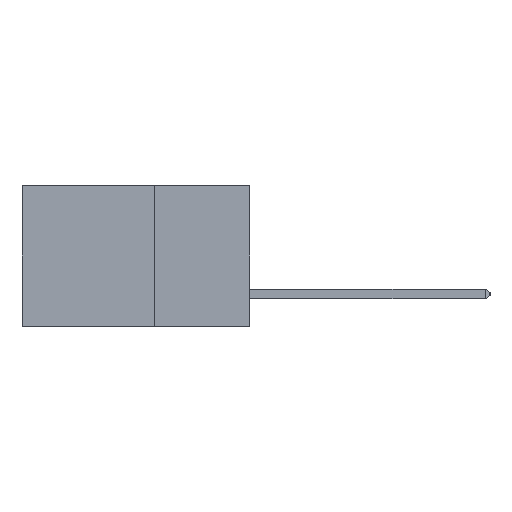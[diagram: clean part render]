
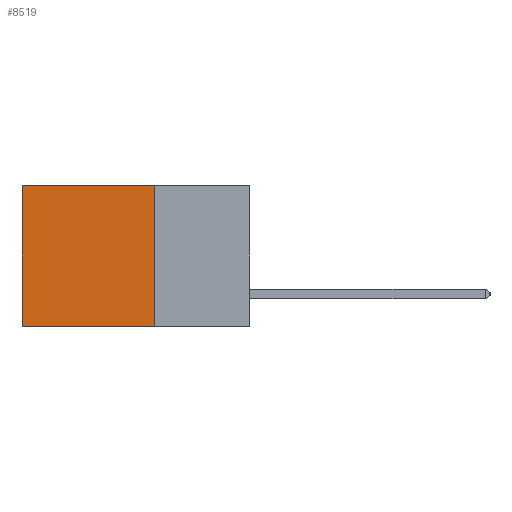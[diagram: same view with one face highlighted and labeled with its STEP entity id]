
A CAD part, left-side view. The second image highlights one B-rep face of the part: STEP entity #8519.
In plain terms, the highlighted planar face has unit normal (-1, 0, 0).
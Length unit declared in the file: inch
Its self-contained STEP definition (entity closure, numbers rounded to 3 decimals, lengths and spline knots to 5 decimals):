
#1531 = DIRECTION ( 'NONE',  ( 0., 0., -1. ) ) ;
#2820 = ORIENTED_EDGE ( 'NONE', *, *, #31856, .T. ) ;
#3117 = DIRECTION ( 'NONE',  ( 0., 1., 0. ) ) ;
#3577 = LINE ( 'NONE', #36829, #6129 ) ;
#3712 = DIRECTION ( 'NONE',  ( 0., 0., -1. ) ) ;
#5119 = DIRECTION ( 'NONE',  ( 0., 0., -1. ) ) ;
#5290 = EDGE_CURVE ( 'NONE', #38703, #34493, #7250, .T. ) ;
#6129 = VECTOR ( 'NONE', #32997, 39.37008 ) ;
#6438 = VERTEX_POINT ( 'NONE', #40004 ) ;
#7250 = LINE ( 'NONE', #19268, #40865 ) ;
#8394 = CARTESIAN_POINT ( 'NONE',  ( 0.2875, 0.6, 0. ) ) ;
#8519 = ADVANCED_FACE ( 'NONE', ( #40928 ), #27375, .F. ) ;
#10884 = VECTOR ( 'NONE', #3712, 39.37008 ) ;
#11191 = CARTESIAN_POINT ( 'NONE',  ( 0.2875, 0.25, 0. ) ) ;
#12404 = LINE ( 'NONE', #36567, #10884 ) ;
#15074 = EDGE_CURVE ( 'NONE', #6438, #39119, #3577, .T. ) ;
#15323 = LINE ( 'NONE', #24394, #40306 ) ;
#19268 = CARTESIAN_POINT ( 'NONE',  ( 0.2875, 0.25, -0.37 ) ) ;
#24394 = CARTESIAN_POINT ( 'NONE',  ( 0.2875, 0.6, 0. ) ) ;
#25441 = CARTESIAN_POINT ( 'NONE',  ( 0.2875, 0.25, -0.37 ) ) ;
#26002 = ORIENTED_EDGE ( 'NONE', *, *, #15074, .T. ) ;
#27375 = PLANE ( 'NONE',  #34944 ) ;
#31313 = CARTESIAN_POINT ( 'NONE',  ( 0.2875, 0.6, -0.37 ) ) ;
#31856 = EDGE_CURVE ( 'NONE', #39119, #34493, #15323, .T. ) ;
#32197 = ORIENTED_EDGE ( 'NONE', *, *, #5290, .F. ) ;
#32997 = DIRECTION ( 'NONE',  ( 0., 1., 0. ) ) ;
#34493 = VERTEX_POINT ( 'NONE', #31313 ) ;
#34944 = AXIS2_PLACEMENT_3D ( 'NONE', #11191, #40506, #1531 ) ;
#36282 = EDGE_CURVE ( 'NONE', #6438, #38703, #12404, .T. ) ;
#36481 = EDGE_LOOP ( 'NONE', ( #2820, #32197, #39844, #26002 ) ) ;
#36567 = CARTESIAN_POINT ( 'NONE',  ( 0.2875, 0.25, 0. ) ) ;
#36829 = CARTESIAN_POINT ( 'NONE',  ( 0.2875, 0.25, 0. ) ) ;
#38703 = VERTEX_POINT ( 'NONE', #25441 ) ;
#39119 = VERTEX_POINT ( 'NONE', #8394 ) ;
#39844 = ORIENTED_EDGE ( 'NONE', *, *, #36282, .F. ) ;
#40004 = CARTESIAN_POINT ( 'NONE',  ( 0.2875, 0.25, 0. ) ) ;
#40306 = VECTOR ( 'NONE', #5119, 39.37008 ) ;
#40506 = DIRECTION ( 'NONE',  ( 1., 0., 0. ) ) ;
#40865 = VECTOR ( 'NONE', #3117, 39.37008 ) ;
#40928 = FACE_OUTER_BOUND ( 'NONE', #36481, .T. ) ;
